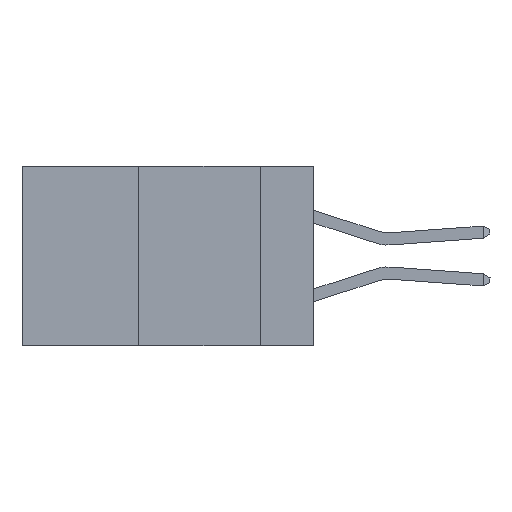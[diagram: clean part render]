
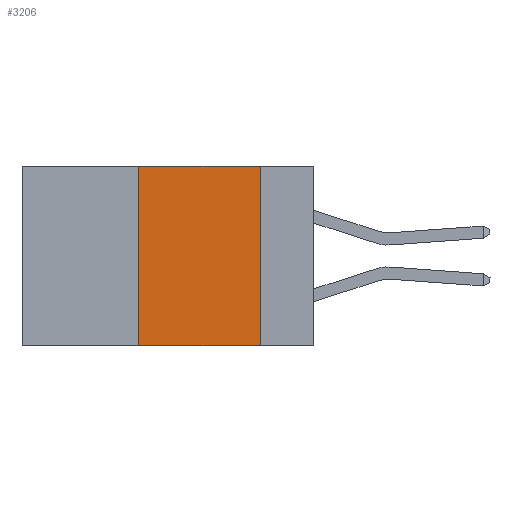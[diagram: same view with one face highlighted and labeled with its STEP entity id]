
A CAD part, left-side view. The second image highlights one B-rep face of the part: STEP entity #3206.
In plain terms, the highlighted planar face has unit normal (-1, 0, 0).
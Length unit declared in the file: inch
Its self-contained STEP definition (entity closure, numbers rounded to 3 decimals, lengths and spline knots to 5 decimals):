
#1155 = CARTESIAN_POINT ( 'NONE',  ( 0., 0.6, 0. ) ) ;
#1638 = LINE ( 'NONE', #8810, #5862 ) ;
#2331 = FACE_OUTER_BOUND ( 'NONE', #15769, .T. ) ;
#2400 = CARTESIAN_POINT ( 'NONE',  ( 0., 0.11, 0. ) ) ;
#3206 = ADVANCED_FACE ( 'NONE', ( #2331 ), #11954, .F. ) ;
#3459 = CARTESIAN_POINT ( 'NONE',  ( 0., 0.36, -0.37 ) ) ;
#3988 = VECTOR ( 'NONE', #9668, 39.37008 ) ;
#5100 = VECTOR ( 'NONE', #20624, 39.37008 ) ;
#5862 = VECTOR ( 'NONE', #19437, 39.37008 ) ;
#5891 = VERTEX_POINT ( 'NONE', #3459 ) ;
#6614 = DIRECTION ( 'NONE',  ( 1., 0., 0. ) ) ;
#6649 = VECTOR ( 'NONE', #18265, 39.37008 ) ;
#7987 = EDGE_CURVE ( 'NONE', #5891, #14036, #20899, .T. ) ;
#8810 = CARTESIAN_POINT ( 'NONE',  ( 0., 0.36, 0. ) ) ;
#9618 = ORIENTED_EDGE ( 'NONE', *, *, #7987, .T. ) ;
#9668 = DIRECTION ( 'NONE',  ( 0., 0., -1. ) ) ;
#9920 = CARTESIAN_POINT ( 'NONE',  ( 0., 0.11, -0.37 ) ) ;
#10270 = EDGE_CURVE ( 'NONE', #5891, #19691, #1638, .T. ) ;
#11838 = CARTESIAN_POINT ( 'NONE',  ( 0., 0.36, 0. ) ) ;
#11885 = ORIENTED_EDGE ( 'NONE', *, *, #14811, .F. ) ;
#11954 = PLANE ( 'NONE',  #18123 ) ;
#13261 = ORIENTED_EDGE ( 'NONE', *, *, #10270, .F. ) ;
#13569 = LINE ( 'NONE', #2400, #3988 ) ;
#14036 = VERTEX_POINT ( 'NONE', #9920 ) ;
#14427 = EDGE_CURVE ( 'NONE', #15282, #14036, #13569, .T. ) ;
#14687 = LINE ( 'NONE', #18849, #5100 ) ;
#14735 = CARTESIAN_POINT ( 'NONE',  ( 0., 0.11, 0. ) ) ;
#14811 = EDGE_CURVE ( 'NONE', #19691, #15282, #14687, .T. ) ;
#15282 = VERTEX_POINT ( 'NONE', #14735 ) ;
#15769 = EDGE_LOOP ( 'NONE', ( #20125, #11885, #13261, #9618 ) ) ;
#16492 = CARTESIAN_POINT ( 'NONE',  ( 0., 0.6, -0.37 ) ) ;
#18123 = AXIS2_PLACEMENT_3D ( 'NONE', #1155, #6614, #19117 ) ;
#18265 = DIRECTION ( 'NONE',  ( 0., -1., 0. ) ) ;
#18849 = CARTESIAN_POINT ( 'NONE',  ( 0., 0.6, 0. ) ) ;
#19117 = DIRECTION ( 'NONE',  ( 0., 0., -1. ) ) ;
#19437 = DIRECTION ( 'NONE',  ( 0., 0., 1. ) ) ;
#19691 = VERTEX_POINT ( 'NONE', #11838 ) ;
#20125 = ORIENTED_EDGE ( 'NONE', *, *, #14427, .F. ) ;
#20624 = DIRECTION ( 'NONE',  ( 0., -1., 0. ) ) ;
#20899 = LINE ( 'NONE', #16492, #6649 ) ;
